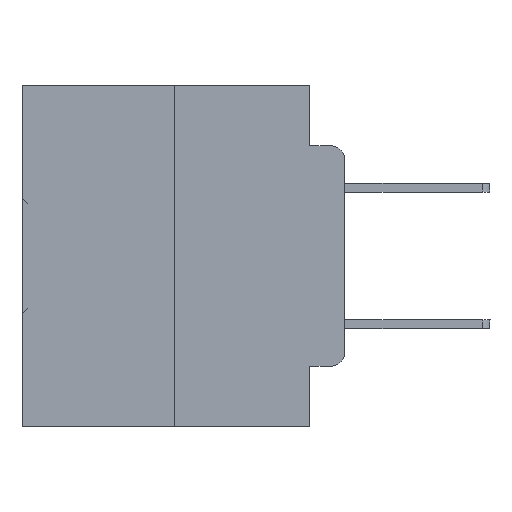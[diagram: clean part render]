
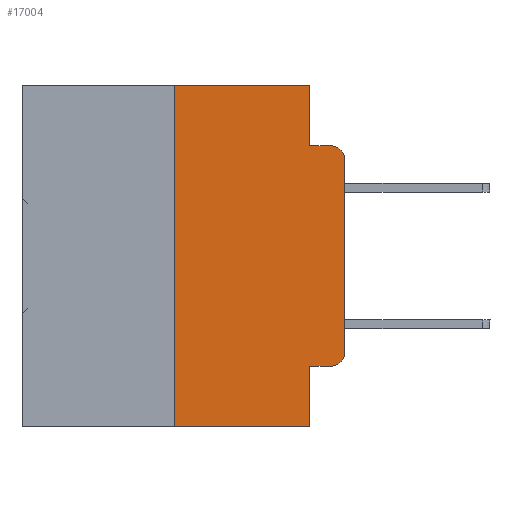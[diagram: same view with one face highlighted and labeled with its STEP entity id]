
A CAD part, left-side view. The second image highlights one B-rep face of the part: STEP entity #17004.
In plain terms, the highlighted planar face has unit normal (-1, 0, 0).
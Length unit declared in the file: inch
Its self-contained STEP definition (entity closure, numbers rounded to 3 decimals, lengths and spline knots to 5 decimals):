
#719 = VECTOR ( 'NONE', #20158, 39.37008 ) ;
#2033 = DIRECTION ( 'NONE',  ( 0., -1., 0. ) ) ;
#2539 = ORIENTED_EDGE ( 'NONE', *, *, #14510, .T. ) ;
#3222 = VERTEX_POINT ( 'NONE', #23065 ) ;
#3503 = CARTESIAN_POINT ( 'NONE',  ( 0., 0.051, -0.0885 ) ) ;
#3940 = DIRECTION ( 'NONE',  ( 0., -1., 0. ) ) ;
#4307 = DIRECTION ( 'NONE',  ( -1., 0., 0. ) ) ;
#5500 = CARTESIAN_POINT ( 'NONE',  ( 0., 0.02, -0.4115 ) ) ;
#6273 = DIRECTION ( 'NONE',  ( 0., 0., -1. ) ) ;
#7560 = CIRCLE ( 'NONE', #9278, 0.02 ) ;
#8032 = EDGE_CURVE ( 'NONE', #29952, #30730, #12628, .T. ) ;
#8272 = ORIENTED_EDGE ( 'NONE', *, *, #31660, .T. ) ;
#8387 = AXIS2_PLACEMENT_3D ( 'NONE', #34243, #25784, #20913 ) ;
#8393 = VERTEX_POINT ( 'NONE', #3503 ) ;
#8490 = DIRECTION ( 'NONE',  ( 0., 0., 1. ) ) ;
#8936 = DIRECTION ( 'NONE',  ( -1., 0., 0. ) ) ;
#9128 = VECTOR ( 'NONE', #13669, 39.37008 ) ;
#9205 = CARTESIAN_POINT ( 'NONE',  ( 0., 0.051, -0.0885 ) ) ;
#9246 = CARTESIAN_POINT ( 'NONE',  ( 0., 0.051, -0.4115 ) ) ;
#9278 = AXIS2_PLACEMENT_3D ( 'NONE', #22958, #4307, #34462 ) ;
#9666 = ORIENTED_EDGE ( 'NONE', *, *, #23249, .T. ) ;
#10241 = CARTESIAN_POINT ( 'NONE',  ( 0., 0.473, 0. ) ) ;
#10617 = LINE ( 'NONE', #24811, #9128 ) ;
#12290 = VECTOR ( 'NONE', #29326, 39.37008 ) ;
#12628 = LINE ( 'NONE', #23575, #12290 ) ;
#12779 = ORIENTED_EDGE ( 'NONE', *, *, #8032, .F. ) ;
#13362 = EDGE_CURVE ( 'NONE', #32911, #21205, #14418, .T. ) ;
#13669 = DIRECTION ( 'NONE',  ( 0., 0., -1. ) ) ;
#14418 = CIRCLE ( 'NONE', #19577, 0.02 ) ;
#14510 = EDGE_CURVE ( 'NONE', #29952, #3222, #17403, .T. ) ;
#14625 = LINE ( 'NONE', #9246, #31500 ) ;
#14843 = PLANE ( 'NONE',  #8387 ) ;
#15045 = CARTESIAN_POINT ( 'NONE',  ( 0., 0.02, -0.1085 ) ) ;
#15189 = FACE_OUTER_BOUND ( 'NONE', #32511, .T. ) ;
#15210 = CARTESIAN_POINT ( 'NONE',  ( 0., 0.473, -0.5 ) ) ;
#15414 = CARTESIAN_POINT ( 'NONE',  ( 0., 0., -0.1085 ) ) ;
#15715 = ORIENTED_EDGE ( 'NONE', *, *, #13362, .T. ) ;
#15760 = EDGE_CURVE ( 'NONE', #30730, #18167, #32337, .T. ) ;
#16534 = VECTOR ( 'NONE', #35221, 39.37008 ) ;
#17004 = ADVANCED_FACE ( 'NONE', ( #15189 ), #14843, .F. ) ;
#17403 = LINE ( 'NONE', #15210, #25370 ) ;
#18167 = VERTEX_POINT ( 'NONE', #32552 ) ;
#18755 = VECTOR ( 'NONE', #8490, 39.37008 ) ;
#18995 = CARTESIAN_POINT ( 'NONE',  ( 0., 0.25, -0.5 ) ) ;
#19094 = ORIENTED_EDGE ( 'NONE', *, *, #21091, .F. ) ;
#19577 = AXIS2_PLACEMENT_3D ( 'NONE', #15045, #8936, #6273 ) ;
#20158 = DIRECTION ( 'NONE',  ( 0., -1., 0. ) ) ;
#20277 = CARTESIAN_POINT ( 'NONE',  ( 0., 0., 0. ) ) ;
#20711 = DIRECTION ( 'NONE',  ( 0., -1., 0. ) ) ;
#20913 = DIRECTION ( 'NONE',  ( 0., 0., -1. ) ) ;
#21023 = CARTESIAN_POINT ( 'NONE',  ( 0., 0.25, 0. ) ) ;
#21091 = EDGE_CURVE ( 'NONE', #18167, #8393, #32519, .T. ) ;
#21205 = VERTEX_POINT ( 'NONE', #21537 ) ;
#21447 = EDGE_CURVE ( 'NONE', #29979, #32911, #30407, .T. ) ;
#21537 = CARTESIAN_POINT ( 'NONE',  ( 0., 0.02, -0.0885 ) ) ;
#22958 = CARTESIAN_POINT ( 'NONE',  ( 0., 0.02, -0.3915 ) ) ;
#23065 = CARTESIAN_POINT ( 'NONE',  ( 0., 0.051, -0.5 ) ) ;
#23187 = LINE ( 'NONE', #9205, #719 ) ;
#23249 = EDGE_CURVE ( 'NONE', #28992, #31798, #14625, .T. ) ;
#23450 = EDGE_CURVE ( 'NONE', #28992, #3222, #10617, .T. ) ;
#23575 = CARTESIAN_POINT ( 'NONE',  ( 0., 0.25, 0. ) ) ;
#23694 = ORIENTED_EDGE ( 'NONE', *, *, #23450, .F. ) ;
#24349 = CARTESIAN_POINT ( 'NONE',  ( 0., 0., -0.3915 ) ) ;
#24811 = CARTESIAN_POINT ( 'NONE',  ( 0., 0.051, 0. ) ) ;
#25370 = VECTOR ( 'NONE', #3940, 39.37008 ) ;
#25784 = DIRECTION ( 'NONE',  ( 1., 0., 0. ) ) ;
#25932 = CARTESIAN_POINT ( 'NONE',  ( 0., 0.051, -0.4115 ) ) ;
#26583 = CARTESIAN_POINT ( 'NONE',  ( 0., 0.051, 0. ) ) ;
#27822 = VECTOR ( 'NONE', #2033, 39.37008 ) ;
#28651 = ORIENTED_EDGE ( 'NONE', *, *, #15760, .F. ) ;
#28992 = VERTEX_POINT ( 'NONE', #25932 ) ;
#29326 = DIRECTION ( 'NONE',  ( 0., 0., 1. ) ) ;
#29633 = EDGE_CURVE ( 'NONE', #8393, #21205, #23187, .T. ) ;
#29952 = VERTEX_POINT ( 'NONE', #18995 ) ;
#29964 = ORIENTED_EDGE ( 'NONE', *, *, #21447, .T. ) ;
#29979 = VERTEX_POINT ( 'NONE', #24349 ) ;
#30407 = LINE ( 'NONE', #20277, #18755 ) ;
#30730 = VERTEX_POINT ( 'NONE', #21023 ) ;
#31500 = VECTOR ( 'NONE', #20711, 39.37008 ) ;
#31660 = EDGE_CURVE ( 'NONE', #31798, #29979, #7560, .T. ) ;
#31798 = VERTEX_POINT ( 'NONE', #5500 ) ;
#32337 = LINE ( 'NONE', #10241, #27822 ) ;
#32511 = EDGE_LOOP ( 'NONE', ( #29964, #15715, #33665, #19094, #28651, #12779, #2539, #23694, #9666, #8272 ) ) ;
#32519 = LINE ( 'NONE', #26583, #16534 ) ;
#32552 = CARTESIAN_POINT ( 'NONE',  ( 0., 0.051, 0. ) ) ;
#32911 = VERTEX_POINT ( 'NONE', #15414 ) ;
#33665 = ORIENTED_EDGE ( 'NONE', *, *, #29633, .F. ) ;
#34243 = CARTESIAN_POINT ( 'NONE',  ( 0., 0.473, 0. ) ) ;
#34462 = DIRECTION ( 'NONE',  ( 0., 0., -1. ) ) ;
#35221 = DIRECTION ( 'NONE',  ( 0., 0., -1. ) ) ;
